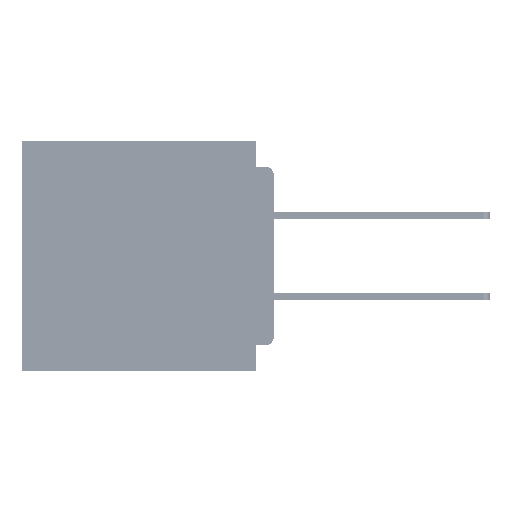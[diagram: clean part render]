
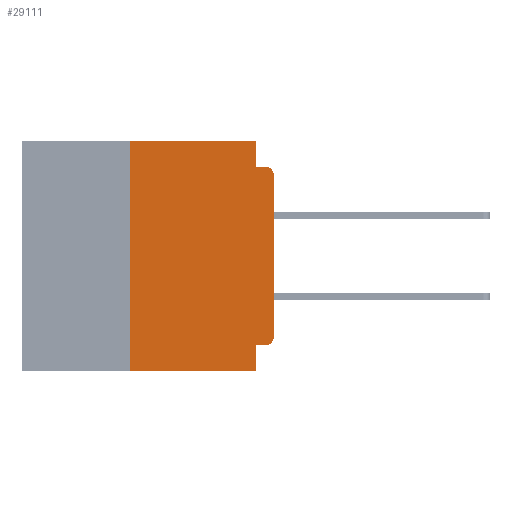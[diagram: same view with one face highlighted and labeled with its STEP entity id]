
A CAD part, left-side view. The second image highlights one B-rep face of the part: STEP entity #29111.
In plain terms, the highlighted planar face has unit normal (-1, 0, 0).
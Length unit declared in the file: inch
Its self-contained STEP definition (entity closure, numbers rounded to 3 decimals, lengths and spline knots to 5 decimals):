
#1701 = LINE ( 'NONE', #4707, #28904 ) ;
#2243 = AXIS2_PLACEMENT_3D ( 'NONE', #8917, #46887, #14394 ) ;
#4292 = VERTEX_POINT ( 'NONE', #22285 ) ;
#4707 = CARTESIAN_POINT ( 'NONE',  ( 0., 0., 0. ) ) ;
#5565 = AXIS2_PLACEMENT_3D ( 'NONE', #16236, #54140, #21702 ) ;
#5626 = ORIENTED_EDGE ( 'NONE', *, *, #34020, .F. ) ;
#5664 = VECTOR ( 'NONE', #65511, 39.37008 ) ;
#6804 = DIRECTION ( 'NONE',  ( 0., -1., 0. ) ) ;
#6916 = VERTEX_POINT ( 'NONE', #44272 ) ;
#7771 = CIRCLE ( 'NONE', #5565, 0.015 ) ;
#8616 = VERTEX_POINT ( 'NONE', #35940 ) ;
#8648 = ORIENTED_EDGE ( 'NONE', *, *, #22882, .F. ) ;
#8917 = CARTESIAN_POINT ( 'NONE',  ( 0., 0.015, -0.06 ) ) ;
#9230 = ORIENTED_EDGE ( 'NONE', *, *, #52507, .F. ) ;
#10404 = LINE ( 'NONE', #56193, #41030 ) ;
#10581 = ORIENTED_EDGE ( 'NONE', *, *, #32126, .T. ) ;
#12259 = CARTESIAN_POINT ( 'NONE',  ( 0., 0.437, 0. ) ) ;
#12302 = ORIENTED_EDGE ( 'NONE', *, *, #13516, .F. ) ;
#12789 = ORIENTED_EDGE ( 'NONE', *, *, #13299, .T. ) ;
#13299 = EDGE_CURVE ( 'NONE', #8616, #6916, #1701, .T. ) ;
#13516 = EDGE_CURVE ( 'NONE', #60764, #24432, #56830, .T. ) ;
#13584 = VECTOR ( 'NONE', #6804, 39.37008 ) ;
#13771 = LINE ( 'NONE', #42638, #51931 ) ;
#14394 = DIRECTION ( 'NONE',  ( 0., 0., -1. ) ) ;
#14611 = CARTESIAN_POINT ( 'NONE',  ( 0., 0.25, -0.4 ) ) ;
#14869 = PLANE ( 'NONE',  #35038 ) ;
#16236 = CARTESIAN_POINT ( 'NONE',  ( 0., 0.015, -0.34 ) ) ;
#16632 = DIRECTION ( 'NONE',  ( 0., 0., 1. ) ) ;
#18920 = VERTEX_POINT ( 'NONE', #28019 ) ;
#19036 = CARTESIAN_POINT ( 'NONE',  ( 0., 0.031, -0.045 ) ) ;
#19110 = EDGE_CURVE ( 'NONE', #36464, #43925, #10404, .T. ) ;
#21702 = DIRECTION ( 'NONE',  ( 0., 0., -1. ) ) ;
#22114 = ORIENTED_EDGE ( 'NONE', *, *, #55435, .F. ) ;
#22285 = CARTESIAN_POINT ( 'NONE',  ( 0., 0.015, -0.355 ) ) ;
#22882 = EDGE_CURVE ( 'NONE', #24432, #36464, #44877, .T. ) ;
#24432 = VERTEX_POINT ( 'NONE', #34031 ) ;
#25681 = DIRECTION ( 'NONE',  ( 0., 0., -1. ) ) ;
#25790 = DIRECTION ( 'NONE',  ( 1., 0., 0. ) ) ;
#26282 = VERTEX_POINT ( 'NONE', #63965 ) ;
#26599 = VECTOR ( 'NONE', #16632, 39.37008 ) ;
#27796 = CIRCLE ( 'NONE', #2243, 0.015 ) ;
#28019 = CARTESIAN_POINT ( 'NONE',  ( 0., 0.031, -0.355 ) ) ;
#28904 = VECTOR ( 'NONE', #53330, 39.37008 ) ;
#29036 = EDGE_CURVE ( 'NONE', #6916, #43925, #27796, .T. ) ;
#29111 = ADVANCED_FACE ( 'NONE', ( #38850 ), #14869, .F. ) ;
#30920 = CARTESIAN_POINT ( 'NONE',  ( 0., 0.031, 0. ) ) ;
#31128 = CARTESIAN_POINT ( 'NONE',  ( 0., 0.015, -0.045 ) ) ;
#32126 = EDGE_CURVE ( 'NONE', #4292, #8616, #7771, .T. ) ;
#34020 = EDGE_CURVE ( 'NONE', #52442, #60764, #41076, .T. ) ;
#34031 = CARTESIAN_POINT ( 'NONE',  ( 0., 0.031, 0. ) ) ;
#35038 = AXIS2_PLACEMENT_3D ( 'NONE', #58240, #25790, #63657 ) ;
#35153 = CARTESIAN_POINT ( 'NONE',  ( 0., 0.25, 0. ) ) ;
#35940 = CARTESIAN_POINT ( 'NONE',  ( 0., 0., -0.34 ) ) ;
#36050 = CARTESIAN_POINT ( 'NONE',  ( 0., 0.437, -0.4 ) ) ;
#36464 = VERTEX_POINT ( 'NONE', #19036 ) ;
#37127 = EDGE_CURVE ( 'NONE', #52442, #26282, #64236, .T. ) ;
#38251 = CARTESIAN_POINT ( 'NONE',  ( 0., 0.25, -0.4 ) ) ;
#38850 = FACE_OUTER_BOUND ( 'NONE', #69285, .T. ) ;
#41030 = VECTOR ( 'NONE', #50970, 39.37008 ) ;
#41076 = LINE ( 'NONE', #38251, #26599 ) ;
#41148 = ORIENTED_EDGE ( 'NONE', *, *, #37127, .T. ) ;
#41524 = VECTOR ( 'NONE', #25681, 39.37008 ) ;
#42638 = CARTESIAN_POINT ( 'NONE',  ( 0., 0., -0.355 ) ) ;
#43925 = VERTEX_POINT ( 'NONE', #31128 ) ;
#44043 = CARTESIAN_POINT ( 'NONE',  ( 0., 0.031, -0.4 ) ) ;
#44272 = CARTESIAN_POINT ( 'NONE',  ( 0., 0., -0.06 ) ) ;
#44877 = LINE ( 'NONE', #30920, #41524 ) ;
#46887 = DIRECTION ( 'NONE',  ( -1., 0., 0. ) ) ;
#49307 = ORIENTED_EDGE ( 'NONE', *, *, #19110, .F. ) ;
#49859 = VECTOR ( 'NONE', #52341, 39.37008 ) ;
#50639 = LINE ( 'NONE', #44043, #5664 ) ;
#50970 = DIRECTION ( 'NONE',  ( 0., -1., 0. ) ) ;
#51931 = VECTOR ( 'NONE', #69537, 39.37008 ) ;
#52341 = DIRECTION ( 'NONE',  ( 0., -1., 0. ) ) ;
#52442 = VERTEX_POINT ( 'NONE', #14611 ) ;
#52507 = EDGE_CURVE ( 'NONE', #4292, #18920, #13771, .T. ) ;
#53330 = DIRECTION ( 'NONE',  ( 0., 0., 1. ) ) ;
#54140 = DIRECTION ( 'NONE',  ( -1., 0., 0. ) ) ;
#55435 = EDGE_CURVE ( 'NONE', #18920, #26282, #50639, .T. ) ;
#56193 = CARTESIAN_POINT ( 'NONE',  ( 0., 0., -0.045 ) ) ;
#56830 = LINE ( 'NONE', #12259, #13584 ) ;
#58240 = CARTESIAN_POINT ( 'NONE',  ( 0., 0.437, 0. ) ) ;
#60764 = VERTEX_POINT ( 'NONE', #35153 ) ;
#63657 = DIRECTION ( 'NONE',  ( 0., 0., -1. ) ) ;
#63965 = CARTESIAN_POINT ( 'NONE',  ( 0., 0.031, -0.4 ) ) ;
#64161 = ORIENTED_EDGE ( 'NONE', *, *, #29036, .T. ) ;
#64236 = LINE ( 'NONE', #36050, #49859 ) ;
#65511 = DIRECTION ( 'NONE',  ( 0., 0., -1. ) ) ;
#69285 = EDGE_LOOP ( 'NONE', ( #12789, #64161, #49307, #8648, #12302, #5626, #41148, #22114, #9230, #10581 ) ) ;
#69537 = DIRECTION ( 'NONE',  ( 0., 1., 0. ) ) ;
